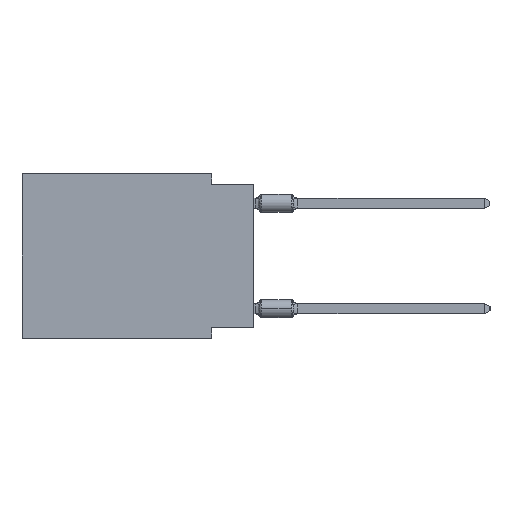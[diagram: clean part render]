
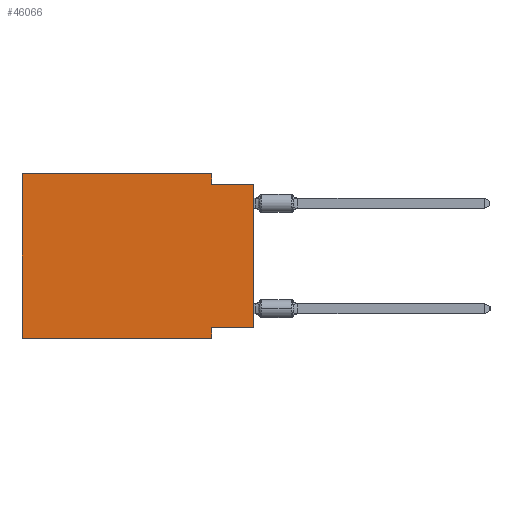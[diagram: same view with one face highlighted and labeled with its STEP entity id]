
A CAD part, left-side view. The second image highlights one B-rep face of the part: STEP entity #46066.
In plain terms, the highlighted planar face has unit normal (-1, 0, 0).
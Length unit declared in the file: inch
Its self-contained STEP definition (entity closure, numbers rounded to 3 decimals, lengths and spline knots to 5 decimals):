
#140 = ORIENTED_EDGE ( 'NONE', *, *, #36517, .T. ) ;
#949 = PLANE ( 'NONE',  #7956 ) ;
#996 = VERTEX_POINT ( 'NONE', #11661 ) ;
#1224 = ORIENTED_EDGE ( 'NONE', *, *, #1832, .F. ) ;
#1832 = EDGE_CURVE ( 'NONE', #20515, #12762, #26867, .T. ) ;
#3126 = CARTESIAN_POINT ( 'NONE',  ( 0., 0.55, 0. ) ) ;
#3462 = EDGE_CURVE ( 'NONE', #14737, #43962, #6662, .T. ) ;
#6031 = CARTESIAN_POINT ( 'NONE',  ( 0., 0., -0.365 ) ) ;
#6662 = LINE ( 'NONE', #3126, #40140 ) ;
#7534 = CARTESIAN_POINT ( 'NONE',  ( 0., 0.1, -0.025 ) ) ;
#7956 = AXIS2_PLACEMENT_3D ( 'NONE', #15558, #36563, #8017 ) ;
#8017 = DIRECTION ( 'NONE',  ( 0., 0., -1. ) ) ;
#9406 = CARTESIAN_POINT ( 'NONE',  ( 0., 0., -0.025 ) ) ;
#10248 = LINE ( 'NONE', #6031, #26973 ) ;
#10318 = VECTOR ( 'NONE', #44126, 39.37008 ) ;
#10482 = DIRECTION ( 'NONE',  ( 0., 0., -1. ) ) ;
#11157 = VECTOR ( 'NONE', #10482, 39.37008 ) ;
#11661 = CARTESIAN_POINT ( 'NONE',  ( 0., 0.1, -0.365 ) ) ;
#12497 = ORIENTED_EDGE ( 'NONE', *, *, #3462, .F. ) ;
#12762 = VERTEX_POINT ( 'NONE', #28115 ) ;
#13135 = VECTOR ( 'NONE', #29180, 39.37008 ) ;
#13408 = ORIENTED_EDGE ( 'NONE', *, *, #19090, .T. ) ;
#14087 = EDGE_CURVE ( 'NONE', #996, #18874, #29972, .T. ) ;
#14549 = LINE ( 'NONE', #39551, #39961 ) ;
#14737 = VERTEX_POINT ( 'NONE', #22773 ) ;
#15253 = CARTESIAN_POINT ( 'NONE',  ( 0., 0.55, 0. ) ) ;
#15558 = CARTESIAN_POINT ( 'NONE',  ( 0., 0.55, 0. ) ) ;
#15793 = DIRECTION ( 'NONE',  ( 0., -1., 0. ) ) ;
#17730 = DIRECTION ( 'NONE',  ( 0., -1., 0. ) ) ;
#18641 = CARTESIAN_POINT ( 'NONE',  ( 0., 0., -0.365 ) ) ;
#18809 = LINE ( 'NONE', #15253, #13135 ) ;
#18874 = VERTEX_POINT ( 'NONE', #30850 ) ;
#19090 = EDGE_CURVE ( 'NONE', #20518, #12762, #14549, .T. ) ;
#19719 = EDGE_LOOP ( 'NONE', ( #13408, #1224, #27417, #12497, #45708, #140, #45586, #28875 ) ) ;
#20515 = VERTEX_POINT ( 'NONE', #7534 ) ;
#20518 = VERTEX_POINT ( 'NONE', #18641 ) ;
#22773 = CARTESIAN_POINT ( 'NONE',  ( 0., 0.55, 0. ) ) ;
#23122 = LINE ( 'NONE', #23580, #35409 ) ;
#23339 = DIRECTION ( 'NONE',  ( 0., -1., 0. ) ) ;
#23580 = CARTESIAN_POINT ( 'NONE',  ( 0., 0.55, -0.39 ) ) ;
#26098 = CARTESIAN_POINT ( 'NONE',  ( 0., 0.55, -0.39 ) ) ;
#26867 = LINE ( 'NONE', #9406, #35202 ) ;
#26973 = VECTOR ( 'NONE', #41866, 39.37008 ) ;
#27417 = ORIENTED_EDGE ( 'NONE', *, *, #32949, .F. ) ;
#28115 = CARTESIAN_POINT ( 'NONE',  ( 0., 0., -0.025 ) ) ;
#28171 = CARTESIAN_POINT ( 'NONE',  ( 0., 0.1, 0. ) ) ;
#28875 = ORIENTED_EDGE ( 'NONE', *, *, #32941, .F. ) ;
#29180 = DIRECTION ( 'NONE',  ( 0., 0., 1. ) ) ;
#29972 = LINE ( 'NONE', #39900, #10318 ) ;
#30850 = CARTESIAN_POINT ( 'NONE',  ( 0., 0.1, -0.39 ) ) ;
#32941 = EDGE_CURVE ( 'NONE', #20518, #996, #10248, .T. ) ;
#32949 = EDGE_CURVE ( 'NONE', #43962, #20515, #42792, .T. ) ;
#35202 = VECTOR ( 'NONE', #23339, 39.37008 ) ;
#35409 = VECTOR ( 'NONE', #15793, 39.37008 ) ;
#36517 = EDGE_CURVE ( 'NONE', #42586, #18874, #23122, .T. ) ;
#36563 = DIRECTION ( 'NONE',  ( 1., 0., 0. ) ) ;
#39551 = CARTESIAN_POINT ( 'NONE',  ( 0., 0., 0. ) ) ;
#39900 = CARTESIAN_POINT ( 'NONE',  ( 0., 0.1, -0.39 ) ) ;
#39961 = VECTOR ( 'NONE', #40018, 39.37008 ) ;
#40018 = DIRECTION ( 'NONE',  ( 0., 0., 1. ) ) ;
#40140 = VECTOR ( 'NONE', #17730, 39.37008 ) ;
#40497 = CARTESIAN_POINT ( 'NONE',  ( 0., 0.1, 0. ) ) ;
#41866 = DIRECTION ( 'NONE',  ( 0., 1., 0. ) ) ;
#42586 = VERTEX_POINT ( 'NONE', #26098 ) ;
#42792 = LINE ( 'NONE', #28171, #11157 ) ;
#43938 = EDGE_CURVE ( 'NONE', #42586, #14737, #18809, .T. ) ;
#43962 = VERTEX_POINT ( 'NONE', #40497 ) ;
#44126 = DIRECTION ( 'NONE',  ( 0., 0., -1. ) ) ;
#44559 = FACE_OUTER_BOUND ( 'NONE', #19719, .T. ) ;
#45586 = ORIENTED_EDGE ( 'NONE', *, *, #14087, .F. ) ;
#45708 = ORIENTED_EDGE ( 'NONE', *, *, #43938, .F. ) ;
#46066 = ADVANCED_FACE ( 'NONE', ( #44559 ), #949, .F. ) ;
